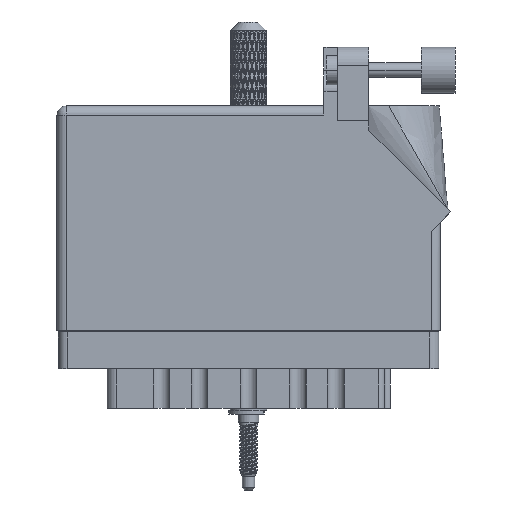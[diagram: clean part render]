
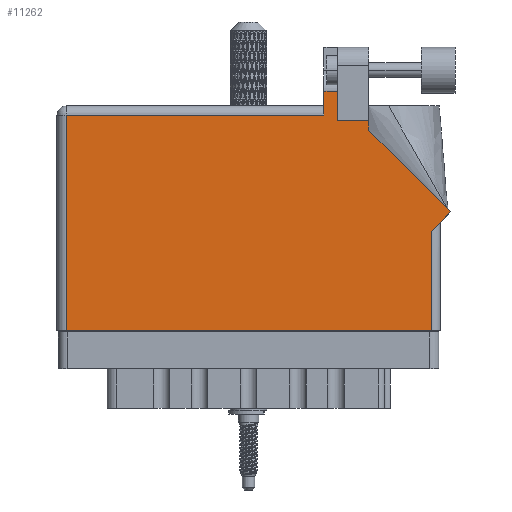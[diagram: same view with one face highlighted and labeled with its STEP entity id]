
A CAD part, front view. The second image highlights one B-rep face of the part: STEP entity #11262.
In plain terms, the highlighted face is planar.
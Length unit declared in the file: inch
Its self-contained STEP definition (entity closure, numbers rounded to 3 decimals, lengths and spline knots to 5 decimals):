
#71 = VECTOR ( 'NONE', #5343, 39.37008 ) ;
#309 = EDGE_CURVE ( 'NONE', #66359, #109608, #58850, .T. ) ;
#1461 = CARTESIAN_POINT ( 'NONE',  ( 1.819, 1.468, 0. ) ) ;
#2687 = DIRECTION ( 'NONE',  ( 0., 0., -1. ) ) ;
#3794 = PLANE ( 'NONE',  #72207 ) ;
#3831 = VERTEX_POINT ( 'NONE', #104941 ) ;
#4204 = VECTOR ( 'NONE', #47254, 39.37008 ) ;
#4319 = VERTEX_POINT ( 'NONE', #63898 ) ;
#5343 = DIRECTION ( 'NONE',  ( 0.707, 0.707, 0. ) ) ;
#6629 = VERTEX_POINT ( 'NONE', #87277 ) ;
#8544 = ORIENTED_EDGE ( 'NONE', *, *, #35661, .T. ) ;
#8990 = DIRECTION ( 'NONE',  ( 0., -1., 0. ) ) ;
#9550 = VECTOR ( 'NONE', #16524, 39.37008 ) ;
#10204 = DIRECTION ( 'NONE',  ( 0., 1., 0. ) ) ;
#11262 = ADVANCED_FACE ( 'NONE', ( #110015 ), #3794, .F. ) ;
#11300 = VECTOR ( 'NONE', #8990, 39.37008 ) ;
#11474 = CARTESIAN_POINT ( 'NONE',  ( 2.55, 0.737, 0. ) ) ;
#11675 = EDGE_CURVE ( 'NONE', #4319, #80191, #29314, .T. ) ;
#12401 = LINE ( 'NONE', #45062, #83324 ) ;
#13068 = CARTESIAN_POINT ( 'NONE',  ( 2.126, 1.36442, 0. ) ) ;
#16524 = DIRECTION ( 'NONE',  ( 0., 1., 0. ) ) ;
#20123 = ORIENTED_EDGE ( 'NONE', *, *, #104885, .T. ) ;
#20685 = CARTESIAN_POINT ( 'NONE',  ( 1.913, 1.43, 0. ) ) ;
#22146 = CARTESIAN_POINT ( 'NONE',  ( 2.55, 0.675, 0. ) ) ;
#23757 = LINE ( 'NONE', #91627, #71 ) ;
#29314 = LINE ( 'NONE', #11474, #4204 ) ;
#29911 = ORIENTED_EDGE ( 'NONE', *, *, #11675, .T. ) ;
#34109 = CARTESIAN_POINT ( 'NONE',  ( 1.819, 1.6315, 0. ) ) ;
#35649 = VERTEX_POINT ( 'NONE', #55197 ) ;
#35661 = EDGE_CURVE ( 'NONE', #6629, #35649, #111310, .T. ) ;
#36210 = ORIENTED_EDGE ( 'NONE', *, *, #56375, .T. ) ;
#36633 = CARTESIAN_POINT ( 'NONE',  ( 1.819, 1.53, 0. ) ) ;
#38293 = VECTOR ( 'NONE', #100512, 39.37008 ) ;
#41284 = EDGE_CURVE ( 'NONE', #35649, #4319, #43842, .T. ) ;
#43786 = LINE ( 'NONE', #86595, #81321 ) ;
#43842 = LINE ( 'NONE', #82622, #38293 ) ;
#45062 = CARTESIAN_POINT ( 'NONE',  ( 2.126, 1.43, 0. ) ) ;
#45830 = CARTESIAN_POINT ( 'NONE',  ( 2.68271, 0.80771, 0. ) ) ;
#47254 = DIRECTION ( 'NONE',  ( 0., 1., 0. ) ) ;
#48186 = CARTESIAN_POINT ( 'NONE',  ( 0.062, 0., 0. ) ) ;
#52149 = ORIENTED_EDGE ( 'NONE', *, *, #41284, .T. ) ;
#55197 = CARTESIAN_POINT ( 'NONE',  ( 0.062, 0., 0. ) ) ;
#56375 = EDGE_CURVE ( 'NONE', #3831, #66359, #12401, .T. ) ;
#57881 = DIRECTION ( 'NONE',  ( -0.707, 0.707, 0. ) ) ;
#58850 = LINE ( 'NONE', #63481, #102015 ) ;
#60557 = CARTESIAN_POINT ( 'NONE',  ( 2.24377, 1.6315, 0. ) ) ;
#61262 = VECTOR ( 'NONE', #92112, 39.37008 ) ;
#63481 = CARTESIAN_POINT ( 'NONE',  ( 1.913, 1.43, 0. ) ) ;
#63898 = CARTESIAN_POINT ( 'NONE',  ( 2.55, 0., 0. ) ) ;
#64259 = ORIENTED_EDGE ( 'NONE', *, *, #95317, .T. ) ;
#65276 = CARTESIAN_POINT ( 'NONE',  ( 2.68271, 0.80771, 0. ) ) ;
#65481 = LINE ( 'NONE', #36633, #11300 ) ;
#65606 = DIRECTION ( 'NONE',  ( -1., 0., 0. ) ) ;
#66359 = VERTEX_POINT ( 'NONE', #20685 ) ;
#70388 = LINE ( 'NONE', #65276, #78907 ) ;
#71230 = VECTOR ( 'NONE', #104856, 39.37008 ) ;
#72207 = AXIS2_PLACEMENT_3D ( 'NONE', #91680, #2687, #65606 ) ;
#75418 = CARTESIAN_POINT ( 'NONE',  ( 1.913, 1.6315, 0. ) ) ;
#76786 = VERTEX_POINT ( 'NONE', #13068 ) ;
#78907 = VECTOR ( 'NONE', #57881, 39.37008 ) ;
#80191 = VERTEX_POINT ( 'NONE', #22146 ) ;
#80259 = ORIENTED_EDGE ( 'NONE', *, *, #100579, .T. ) ;
#80825 = DIRECTION ( 'NONE',  ( -1., 0., 0. ) ) ;
#80941 = VERTEX_POINT ( 'NONE', #34109 ) ;
#81321 = VECTOR ( 'NONE', #95521, 39.37008 ) ;
#82622 = CARTESIAN_POINT ( 'NONE',  ( 0., 0., 0. ) ) ;
#83324 = VECTOR ( 'NONE', #80825, 39.37008 ) ;
#84499 = EDGE_CURVE ( 'NONE', #109608, #80941, #96249, .T. ) ;
#86595 = CARTESIAN_POINT ( 'NONE',  ( 0., 1.468, 0. ) ) ;
#87277 = CARTESIAN_POINT ( 'NONE',  ( 0.062, 1.468, 0. ) ) ;
#91627 = CARTESIAN_POINT ( 'NONE',  ( 2.612, 0.737, 0. ) ) ;
#91680 = CARTESIAN_POINT ( 'NONE',  ( 0., 1.53, 0. ) ) ;
#92112 = DIRECTION ( 'NONE',  ( 0., -1., 0. ) ) ;
#94161 = ORIENTED_EDGE ( 'NONE', *, *, #84499, .T. ) ;
#94312 = ORIENTED_EDGE ( 'NONE', *, *, #110922, .T. ) ;
#94318 = VERTEX_POINT ( 'NONE', #1461 ) ;
#94477 = LINE ( 'NONE', #114397, #9550 ) ;
#95317 = EDGE_CURVE ( 'NONE', #109762, #76786, #70388, .T. ) ;
#95521 = DIRECTION ( 'NONE',  ( -1., 0., 0. ) ) ;
#96249 = LINE ( 'NONE', #60557, #71230 ) ;
#98661 = EDGE_LOOP ( 'NONE', ( #105430, #94161, #80259, #94312, #8544, #52149, #29911, #20123, #64259, #103889, #36210 ) ) ;
#100512 = DIRECTION ( 'NONE',  ( 1., 0., 0. ) ) ;
#100579 = EDGE_CURVE ( 'NONE', #80941, #94318, #65481, .T. ) ;
#102015 = VECTOR ( 'NONE', #10204, 39.37008 ) ;
#103889 = ORIENTED_EDGE ( 'NONE', *, *, #105931, .T. ) ;
#104856 = DIRECTION ( 'NONE',  ( -1., 0., 0. ) ) ;
#104885 = EDGE_CURVE ( 'NONE', #80191, #109762, #23757, .T. ) ;
#104941 = CARTESIAN_POINT ( 'NONE',  ( 2.126, 1.43, 0. ) ) ;
#105430 = ORIENTED_EDGE ( 'NONE', *, *, #309, .T. ) ;
#105931 = EDGE_CURVE ( 'NONE', #76786, #3831, #94477, .T. ) ;
#109608 = VERTEX_POINT ( 'NONE', #75418 ) ;
#109762 = VERTEX_POINT ( 'NONE', #45830 ) ;
#110015 = FACE_OUTER_BOUND ( 'NONE', #98661, .T. ) ;
#110922 = EDGE_CURVE ( 'NONE', #94318, #6629, #43786, .T. ) ;
#111310 = LINE ( 'NONE', #48186, #61262 ) ;
#114397 = CARTESIAN_POINT ( 'NONE',  ( 2.126, 1.36442, 0. ) ) ;
